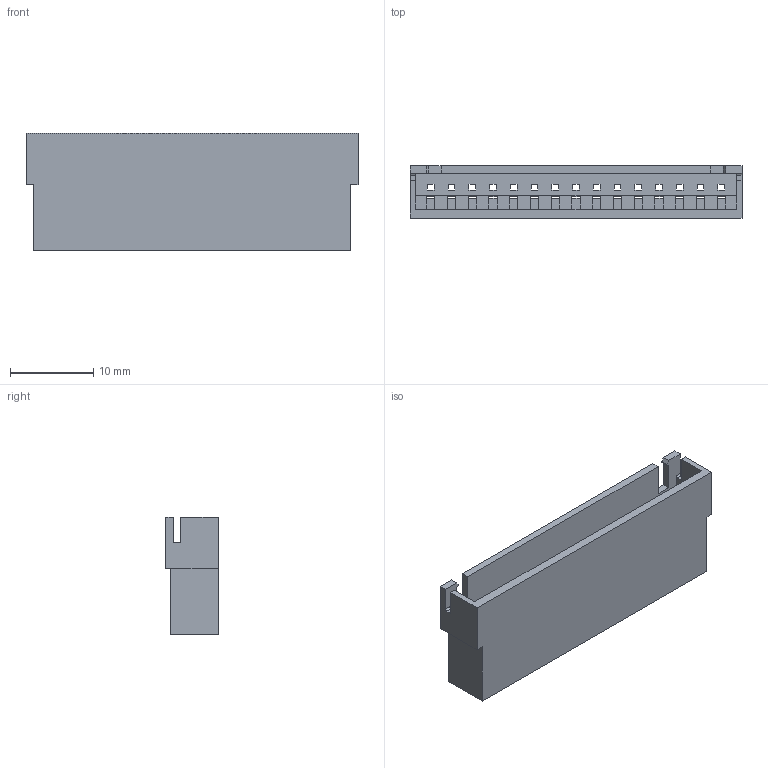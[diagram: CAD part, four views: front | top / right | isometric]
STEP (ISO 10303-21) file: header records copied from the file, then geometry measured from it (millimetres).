
FILE_DESCRIPTION (( 'STEP AP203' ), '1' );
FILE_NAME ('14K-515-210-AA1.STEP', '2024-02-23T14:34:45', ( '' ), ( '' ), 'SwSTEP 2.0', 'SolidWorks 2023', '' );
FILE_SCHEMA (( 'CONFIG_CONTROL_DESIGN' ));
Length unit declared in the file: millimetre
Products named in the file (1): 14K-515-210-AA1
Bounding box: 40 x 6.3 x 14.2 mm (x, y, z)
Volume: 1719.8 mm3; surface area: 3844.3 mm2
Topology: 1 solids, 1 shells, 414 faces, 1248 edges, 822 vertices
Faces by surface type: plane 410, cylinder 4
Entity records: 13877 total; most frequent: ORIENTED_EDGE 2496, CARTESIAN_POINT 2485, DIRECTION 2086, EDGE_CURVE 1248, LINE 1240, VECTOR 1240, VERTEX_POINT 822, EDGE_LOOP 460
